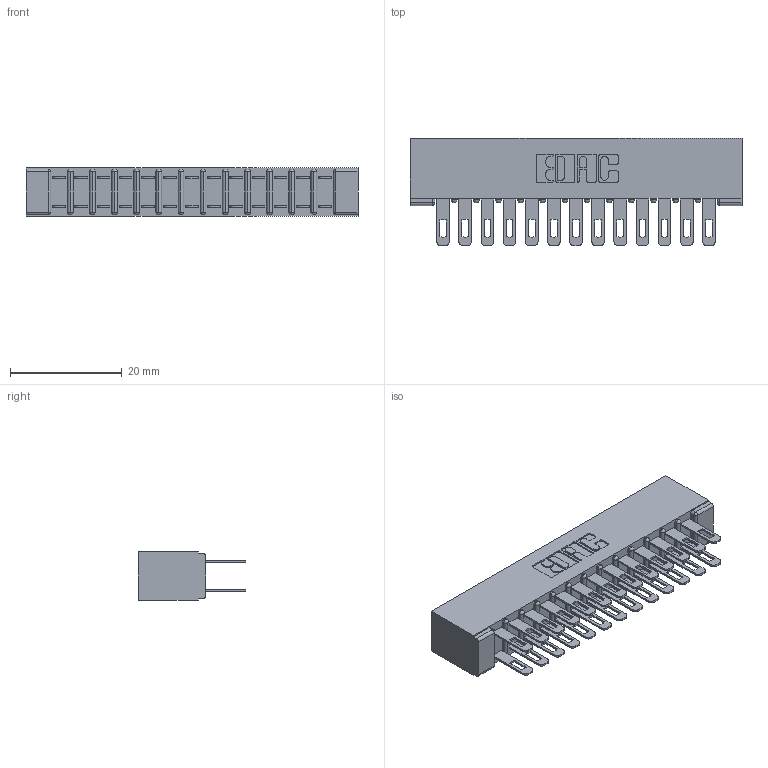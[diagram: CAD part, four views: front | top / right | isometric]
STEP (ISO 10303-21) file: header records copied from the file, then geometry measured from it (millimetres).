
FILE_DESCRIPTION (( 'STEP AP203' ), '1' );
FILE_NAME ('357-026-400-201.STEP', '2020-10-03T01:51:45', ( '' ), ( '' ), 'SwSTEP 2.0', 'SolidWorks 2020', '' );
FILE_SCHEMA (( 'CONFIG_CONTROL_DESIGN' ));
Length unit declared in the file: inch
Products named in the file (3): 307 Part_No Mounting Lugs; 307-290-001_500; 357-026-400-201
Assembly tree (27 placements, depth 2):
  357-026-400-201
    307 Part_No Mounting Lugs
    307-290-001_500  x26
Bounding box: 59.39 x 19.18 x 8.71 mm (x, y, z)
Volume: 4193 mm3; surface area: 7820.6 mm2
Topology: 27 solids, 27 shells, 1320 faces, 3679 edges, 2378 vertices
Faces by surface type: plane 846, cylinder 446, sphere 28
Entity records: 14832 total; most frequent: CARTESIAN_POINT 2429, ORIENTED_EDGE 2402, DIRECTION 2393, EDGE_CURVE 1201, VECTOR 909, LINE 909, VERTEX_POINT 778, AXIS2_PLACEMENT_3D 742
